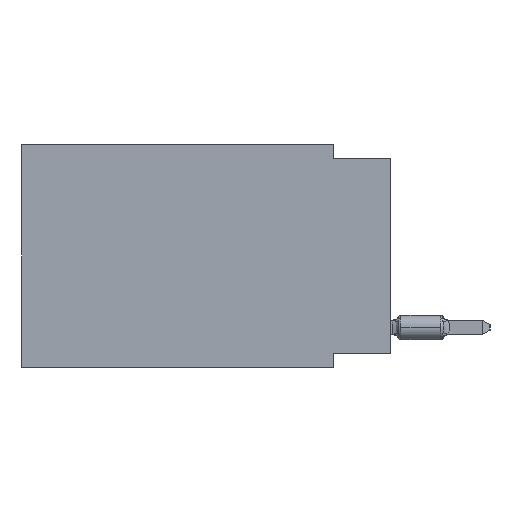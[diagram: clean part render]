
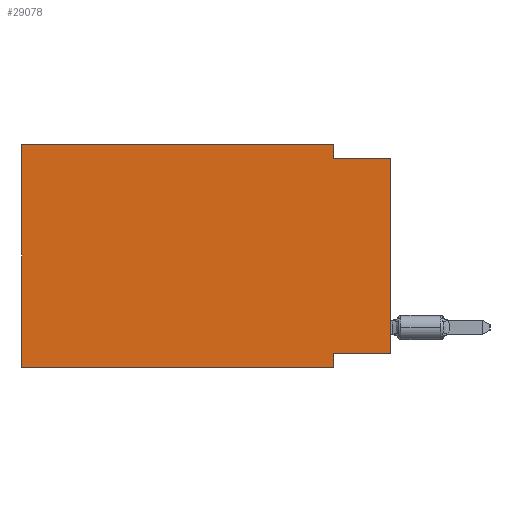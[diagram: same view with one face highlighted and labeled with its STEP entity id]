
A CAD part, left-side view. The second image highlights one B-rep face of the part: STEP entity #29078.
In plain terms, the highlighted planar face has unit normal (-1, 0, 0).
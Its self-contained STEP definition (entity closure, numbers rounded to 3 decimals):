
#723 = ORIENTED_EDGE ( 'NONE', *, *, #31245, .F. ) ;
#1222 = VECTOR ( 'NONE', #8784, 1000. ) ;
#1313 = CARTESIAN_POINT ( 'NONE',  ( 0., 0., -9.271 ) ) ;
#1666 = EDGE_CURVE ( 'NONE', #17464, #6879, #16519, .T. ) ;
#2441 = VERTEX_POINT ( 'NONE', #10919 ) ;
#4095 = EDGE_CURVE ( 'NONE', #41761, #24215, #12628, .T. ) ;
#5151 = EDGE_CURVE ( 'NONE', #16662, #8576, #38747, .T. ) ;
#6145 = CARTESIAN_POINT ( 'NONE',  ( 0., 0., -0.635 ) ) ;
#6873 = CARTESIAN_POINT ( 'NONE',  ( 0., 0., 0. ) ) ;
#6879 = VERTEX_POINT ( 'NONE', #9030 ) ;
#8576 = VERTEX_POINT ( 'NONE', #35422 ) ;
#8784 = DIRECTION ( 'NONE',  ( 0., 0., -1. ) ) ;
#9030 = CARTESIAN_POINT ( 'NONE',  ( 0., 2.54, -0.635 ) ) ;
#10892 = CARTESIAN_POINT ( 'NONE',  ( 0., 2.54, -9.906 ) ) ;
#10919 = CARTESIAN_POINT ( 'NONE',  ( 0., 2.54, -9.271 ) ) ;
#11032 = EDGE_CURVE ( 'NONE', #6879, #8576, #31399, .T. ) ;
#11073 = DIRECTION ( 'NONE',  ( 1., 0., 0. ) ) ;
#12628 = LINE ( 'NONE', #16133, #29493 ) ;
#13549 = CARTESIAN_POINT ( 'NONE',  ( 0., 2.54, 0. ) ) ;
#14427 = CARTESIAN_POINT ( 'NONE',  ( 0., 16.383, 0. ) ) ;
#14525 = ORIENTED_EDGE ( 'NONE', *, *, #1666, .F. ) ;
#15044 = ORIENTED_EDGE ( 'NONE', *, *, #25194, .F. ) ;
#15119 = ORIENTED_EDGE ( 'NONE', *, *, #5151, .T. ) ;
#15128 = CARTESIAN_POINT ( 'NONE',  ( 0., 16.383, 0. ) ) ;
#16133 = CARTESIAN_POINT ( 'NONE',  ( 0., 16.383, -9.906 ) ) ;
#16519 = LINE ( 'NONE', #13549, #1222 ) ;
#16662 = VERTEX_POINT ( 'NONE', #49107 ) ;
#17464 = VERTEX_POINT ( 'NONE', #34166 ) ;
#18821 = CARTESIAN_POINT ( 'NONE',  ( 0., 16.383, 0. ) ) ;
#19964 = AXIS2_PLACEMENT_3D ( 'NONE', #18821, #11073, #39516 ) ;
#21733 = VERTEX_POINT ( 'NONE', #14427 ) ;
#22431 = EDGE_CURVE ( 'NONE', #41761, #21733, #24443, .T. ) ;
#22805 = FACE_OUTER_BOUND ( 'NONE', #22931, .T. ) ;
#22931 = EDGE_LOOP ( 'NONE', ( #15119, #36338, #14525, #723, #44412, #32047, #15044, #29579 ) ) ;
#24215 = VERTEX_POINT ( 'NONE', #42927 ) ;
#24443 = LINE ( 'NONE', #40622, #39883 ) ;
#25194 = EDGE_CURVE ( 'NONE', #2441, #24215, #47554, .T. ) ;
#27397 = DIRECTION ( 'NONE',  ( 0., 0., -1. ) ) ;
#29078 = ADVANCED_FACE ( 'NONE', ( #22805 ), #35552, .F. ) ;
#29493 = VECTOR ( 'NONE', #31841, 1000. ) ;
#29579 = ORIENTED_EDGE ( 'NONE', *, *, #30630, .F. ) ;
#30630 = EDGE_CURVE ( 'NONE', #16662, #2441, #37724, .T. ) ;
#31245 = EDGE_CURVE ( 'NONE', #21733, #17464, #39048, .T. ) ;
#31399 = LINE ( 'NONE', #6145, #32969 ) ;
#31841 = DIRECTION ( 'NONE',  ( 0., -1., 0. ) ) ;
#31940 = CARTESIAN_POINT ( 'NONE',  ( 0., 16.383, -9.906 ) ) ;
#32047 = ORIENTED_EDGE ( 'NONE', *, *, #4095, .T. ) ;
#32574 = DIRECTION ( 'NONE',  ( 0., -1., 0. ) ) ;
#32885 = VECTOR ( 'NONE', #51519, 1000. ) ;
#32969 = VECTOR ( 'NONE', #38561, 1000. ) ;
#33766 = VECTOR ( 'NONE', #43532, 1000. ) ;
#34166 = CARTESIAN_POINT ( 'NONE',  ( 0., 2.54, 0. ) ) ;
#35422 = CARTESIAN_POINT ( 'NONE',  ( 0., 0., -0.635 ) ) ;
#35552 = PLANE ( 'NONE',  #19964 ) ;
#36338 = ORIENTED_EDGE ( 'NONE', *, *, #11032, .F. ) ;
#37724 = LINE ( 'NONE', #1313, #32885 ) ;
#38561 = DIRECTION ( 'NONE',  ( 0., -1., 0. ) ) ;
#38747 = LINE ( 'NONE', #6873, #33766 ) ;
#38889 = VECTOR ( 'NONE', #32574, 1000. ) ;
#39048 = LINE ( 'NONE', #15128, #38889 ) ;
#39516 = DIRECTION ( 'NONE',  ( 0., 0., -1. ) ) ;
#39883 = VECTOR ( 'NONE', #43851, 1000. ) ;
#40622 = CARTESIAN_POINT ( 'NONE',  ( 0., 16.383, 0. ) ) ;
#41761 = VERTEX_POINT ( 'NONE', #31940 ) ;
#42927 = CARTESIAN_POINT ( 'NONE',  ( 0., 2.54, -9.906 ) ) ;
#43532 = DIRECTION ( 'NONE',  ( 0., 0., 1. ) ) ;
#43851 = DIRECTION ( 'NONE',  ( 0., 0., 1. ) ) ;
#44412 = ORIENTED_EDGE ( 'NONE', *, *, #22431, .F. ) ;
#47529 = VECTOR ( 'NONE', #27397, 1000. ) ;
#47554 = LINE ( 'NONE', #10892, #47529 ) ;
#49107 = CARTESIAN_POINT ( 'NONE',  ( 0., 0., -9.271 ) ) ;
#51519 = DIRECTION ( 'NONE',  ( 0., 1., 0. ) ) ;
